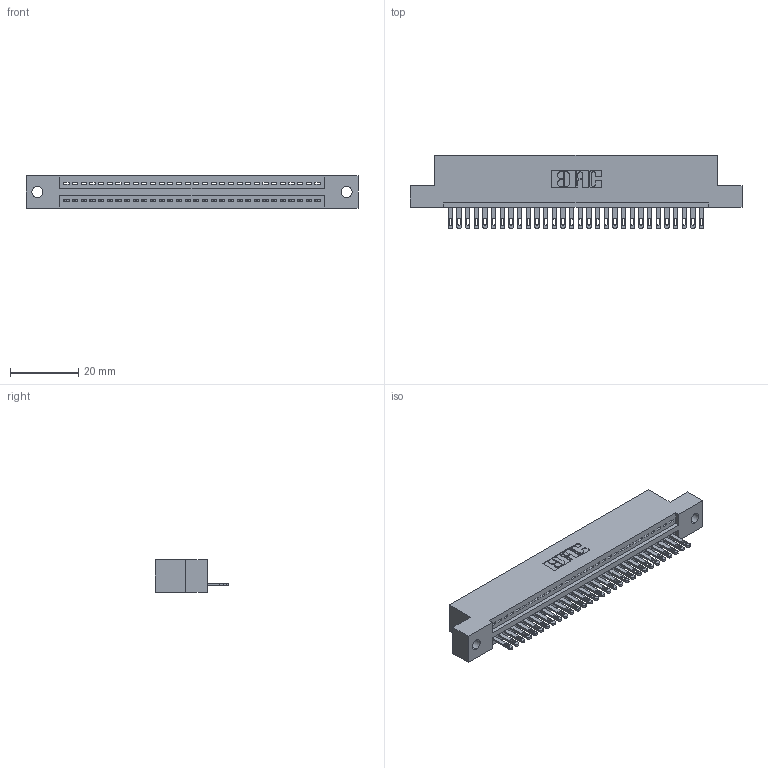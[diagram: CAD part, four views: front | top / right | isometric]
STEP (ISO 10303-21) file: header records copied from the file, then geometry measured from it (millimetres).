
FILE_DESCRIPTION (( 'STEP AP203' ), '1' );
FILE_NAME ('895-030-500-102.STEP', '2020-09-25T17:28:35', ( '' ), ( '' ), 'SwSTEP 2.0', 'SolidWorks 2020', '' );
FILE_SCHEMA (( 'CONFIG_CONTROL_DESIGN' ));
Length unit declared in the file: inch
Products named in the file (3): 895-030-500-102; 345-292-001_345-293-100; 845 Part_Flush Mounting Lugs - 0.128 Dia
Assembly tree (31 placements, depth 2):
  895-030-500-102
    845 Part_Flush Mounting Lugs - 0.128 Dia
    345-292-001_345-293-100  x30
Bounding box: 97.41 x 21.51 x 9.4 mm (x, y, z)
Volume: 9135.6 mm3; surface area: 11773.1 mm2
Topology: 31 solids, 31 shells, 1746 faces, 5381 edges, 3586 vertices
Faces by surface type: plane 1100, cylinder 646
Entity records: 24127 total; most frequent: CARTESIAN_POINT 4186, ORIENTED_EDGE 4150, DIRECTION 3675, EDGE_CURVE 2075, LINE 1819, VECTOR 1819, VERTEX_POINT 1382, AXIS2_PLACEMENT_3D 928
